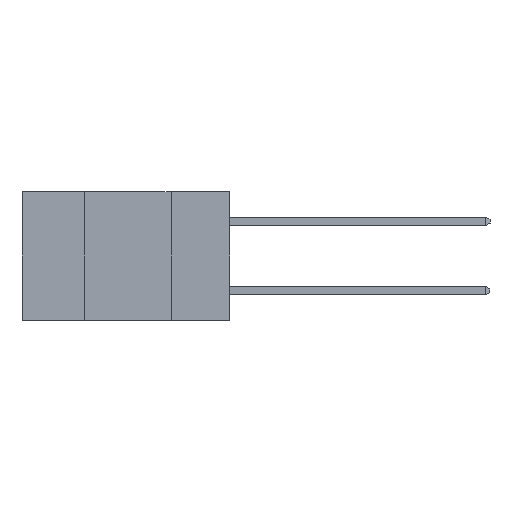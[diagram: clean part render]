
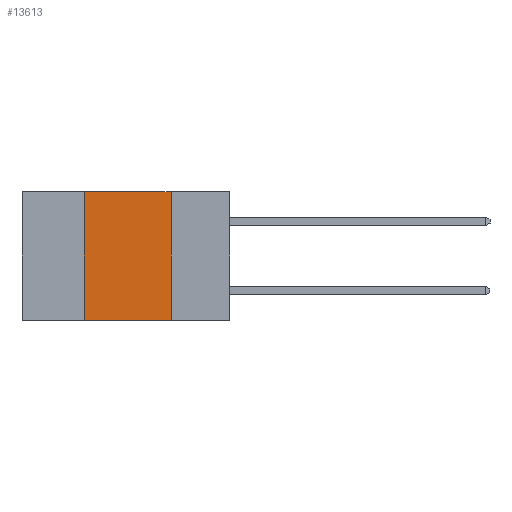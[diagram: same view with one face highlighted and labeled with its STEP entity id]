
A CAD part, left-side view. The second image highlights one B-rep face of the part: STEP entity #13613.
In plain terms, the highlighted planar face has unit normal (-1, 0, 0).
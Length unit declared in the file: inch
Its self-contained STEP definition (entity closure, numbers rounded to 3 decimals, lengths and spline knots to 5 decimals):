
#19 = ORIENTED_EDGE ( 'NONE', *, *, #16067, .F. ) ;
#372 = EDGE_CURVE ( 'NONE', #11817, #4328, #22480, .T. ) ;
#397 = VECTOR ( 'NONE', #11697, 39.37008 ) ;
#1632 = DIRECTION ( 'NONE',  ( 0., 0., -1. ) ) ;
#1709 = CARTESIAN_POINT ( 'NONE',  ( 0., 0.42, 0. ) ) ;
#2013 = CARTESIAN_POINT ( 'NONE',  ( 0., 0.42, -0.37 ) ) ;
#2144 = DIRECTION ( 'NONE',  ( 0., -1., 0. ) ) ;
#2310 = ORIENTED_EDGE ( 'NONE', *, *, #19106, .T. ) ;
#2583 = CARTESIAN_POINT ( 'NONE',  ( 0., 0.42, 0. ) ) ;
#4262 = EDGE_LOOP ( 'NONE', ( #22590, #19, #19608, #2310 ) ) ;
#4328 = VERTEX_POINT ( 'NONE', #1709 ) ;
#4701 = CARTESIAN_POINT ( 'NONE',  ( 0., 0.17, 0. ) ) ;
#5317 = LINE ( 'NONE', #11537, #9540 ) ;
#8075 = CARTESIAN_POINT ( 'NONE',  ( 0., 0.6, -0.37 ) ) ;
#8312 = VECTOR ( 'NONE', #22013, 39.37008 ) ;
#9036 = CARTESIAN_POINT ( 'NONE',  ( 0., 0.17, -0.37 ) ) ;
#9540 = VECTOR ( 'NONE', #9735, 39.37008 ) ;
#9735 = DIRECTION ( 'NONE',  ( 0., 0., -1. ) ) ;
#9875 = VECTOR ( 'NONE', #2144, 39.37008 ) ;
#11095 = FACE_OUTER_BOUND ( 'NONE', #4262, .T. ) ;
#11537 = CARTESIAN_POINT ( 'NONE',  ( 0., 0.17, 0. ) ) ;
#11697 = DIRECTION ( 'NONE',  ( 0., -1., 0. ) ) ;
#11760 = AXIS2_PLACEMENT_3D ( 'NONE', #22907, #12377, #1632 ) ;
#11817 = VERTEX_POINT ( 'NONE', #2013 ) ;
#12377 = DIRECTION ( 'NONE',  ( 1., 0., 0. ) ) ;
#13613 = ADVANCED_FACE ( 'NONE', ( #11095 ), #17669, .F. ) ;
#16067 = EDGE_CURVE ( 'NONE', #4328, #22004, #19340, .T. ) ;
#17669 = PLANE ( 'NONE',  #11760 ) ;
#18322 = LINE ( 'NONE', #8075, #397 ) ;
#19106 = EDGE_CURVE ( 'NONE', #11817, #20143, #18322, .T. ) ;
#19340 = LINE ( 'NONE', #19916, #9875 ) ;
#19608 = ORIENTED_EDGE ( 'NONE', *, *, #372, .F. ) ;
#19916 = CARTESIAN_POINT ( 'NONE',  ( 0., 0.6, 0. ) ) ;
#20143 = VERTEX_POINT ( 'NONE', #9036 ) ;
#21884 = EDGE_CURVE ( 'NONE', #22004, #20143, #5317, .T. ) ;
#22004 = VERTEX_POINT ( 'NONE', #4701 ) ;
#22013 = DIRECTION ( 'NONE',  ( 0., 0., 1. ) ) ;
#22480 = LINE ( 'NONE', #2583, #8312 ) ;
#22590 = ORIENTED_EDGE ( 'NONE', *, *, #21884, .F. ) ;
#22907 = CARTESIAN_POINT ( 'NONE',  ( 0., 0.6, 0. ) ) ;
